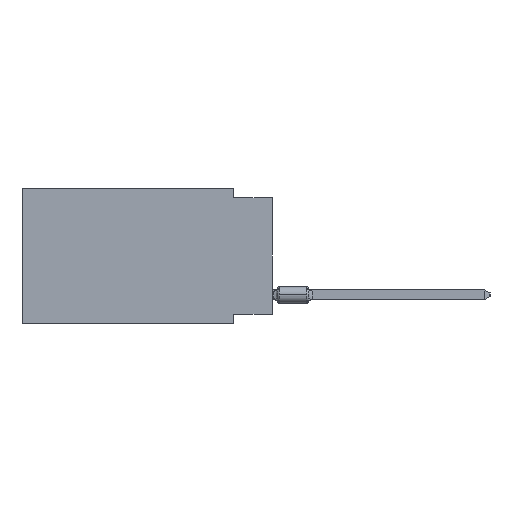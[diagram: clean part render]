
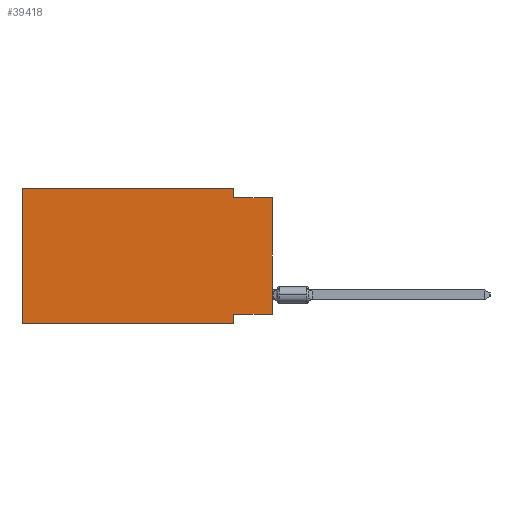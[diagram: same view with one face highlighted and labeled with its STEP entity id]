
A CAD part, left-side view. The second image highlights one B-rep face of the part: STEP entity #39418.
In plain terms, the highlighted planar face has unit normal (-1, 0, 0).
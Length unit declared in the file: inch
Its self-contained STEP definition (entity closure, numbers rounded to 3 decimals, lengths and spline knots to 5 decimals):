
#1447 = VERTEX_POINT ( 'NONE', #66218 ) ;
#1504 = LINE ( 'NONE', #48722, #43938 ) ;
#1848 = FACE_OUTER_BOUND ( 'NONE', #68202, .T. ) ;
#2278 = CARTESIAN_POINT ( 'NONE',  ( 0., 0.645, 0. ) ) ;
#4499 = VECTOR ( 'NONE', #53500, 39.37008 ) ;
#5767 = CARTESIAN_POINT ( 'NONE',  ( 0., 0.1, -0.35 ) ) ;
#6463 = ORIENTED_EDGE ( 'NONE', *, *, #48289, .T. ) ;
#7858 = DIRECTION ( 'NONE',  ( 0., 0., 1. ) ) ;
#8450 = PLANE ( 'NONE',  #67517 ) ;
#8498 = ORIENTED_EDGE ( 'NONE', *, *, #52676, .F. ) ;
#10071 = DIRECTION ( 'NONE',  ( 0., 0., -1. ) ) ;
#10268 = ORIENTED_EDGE ( 'NONE', *, *, #32074, .T. ) ;
#10393 = VERTEX_POINT ( 'NONE', #55037 ) ;
#10540 = VERTEX_POINT ( 'NONE', #61678 ) ;
#10897 = VECTOR ( 'NONE', #47799, 39.37008 ) ;
#11428 = ORIENTED_EDGE ( 'NONE', *, *, #39035, .F. ) ;
#11627 = VECTOR ( 'NONE', #7858, 39.37008 ) ;
#12656 = DIRECTION ( 'NONE',  ( 0., 0., -1. ) ) ;
#13071 = VERTEX_POINT ( 'NONE', #23697 ) ;
#13671 = VERTEX_POINT ( 'NONE', #41412 ) ;
#16174 = LINE ( 'NONE', #58866, #17674 ) ;
#16407 = LINE ( 'NONE', #21311, #4499 ) ;
#17674 = VECTOR ( 'NONE', #25656, 39.37008 ) ;
#18840 = VECTOR ( 'NONE', #66236, 39.37008 ) ;
#21066 = ORIENTED_EDGE ( 'NONE', *, *, #36596, .F. ) ;
#21311 = CARTESIAN_POINT ( 'NONE',  ( 0., 0.645, 0. ) ) ;
#22012 = ORIENTED_EDGE ( 'NONE', *, *, #31696, .F. ) ;
#22060 = VECTOR ( 'NONE', #10071, 39.37008 ) ;
#22874 = LINE ( 'NONE', #61347, #18840 ) ;
#23515 = DIRECTION ( 'NONE',  ( 1., 0., 0. ) ) ;
#23697 = CARTESIAN_POINT ( 'NONE',  ( 0., 0.645, 0. ) ) ;
#25148 = VERTEX_POINT ( 'NONE', #34163 ) ;
#25656 = DIRECTION ( 'NONE',  ( 0., 0., 1. ) ) ;
#26456 = CARTESIAN_POINT ( 'NONE',  ( 0., 0., -0.025 ) ) ;
#27095 = DIRECTION ( 'NONE',  ( 0., 0., -1. ) ) ;
#27178 = CARTESIAN_POINT ( 'NONE',  ( 0., 0.1, 0. ) ) ;
#29430 = CARTESIAN_POINT ( 'NONE',  ( 0., 0.645, 0. ) ) ;
#29437 = EDGE_CURVE ( 'NONE', #10540, #13671, #48176, .T. ) ;
#31696 = EDGE_CURVE ( 'NONE', #33998, #10393, #32355, .T. ) ;
#31703 = LINE ( 'NONE', #26456, #10897 ) ;
#32074 = EDGE_CURVE ( 'NONE', #1447, #40912, #16174, .T. ) ;
#32355 = LINE ( 'NONE', #5767, #36587 ) ;
#32447 = CARTESIAN_POINT ( 'NONE',  ( 0., 0., -0.025 ) ) ;
#33998 = VERTEX_POINT ( 'NONE', #57048 ) ;
#34163 = CARTESIAN_POINT ( 'NONE',  ( 0., 0.645, -0.35 ) ) ;
#36587 = VECTOR ( 'NONE', #27095, 39.37008 ) ;
#36596 = EDGE_CURVE ( 'NONE', #1447, #33998, #1504, .T. ) ;
#39035 = EDGE_CURVE ( 'NONE', #25148, #13071, #55774, .T. ) ;
#39418 = ADVANCED_FACE ( 'NONE', ( #1848 ), #8450, .F. ) ;
#40912 = VERTEX_POINT ( 'NONE', #32447 ) ;
#41412 = CARTESIAN_POINT ( 'NONE',  ( 0., 0.1, -0.025 ) ) ;
#42070 = ORIENTED_EDGE ( 'NONE', *, *, #29437, .F. ) ;
#43938 = VECTOR ( 'NONE', #65517, 39.37008 ) ;
#47799 = DIRECTION ( 'NONE',  ( 0., -1., 0. ) ) ;
#48176 = LINE ( 'NONE', #27178, #22060 ) ;
#48289 = EDGE_CURVE ( 'NONE', #25148, #10393, #22874, .T. ) ;
#48722 = CARTESIAN_POINT ( 'NONE',  ( 0., 0., -0.325 ) ) ;
#52676 = EDGE_CURVE ( 'NONE', #13671, #40912, #31703, .T. ) ;
#53500 = DIRECTION ( 'NONE',  ( 0., -1., 0. ) ) ;
#55037 = CARTESIAN_POINT ( 'NONE',  ( 0., 0.1, -0.35 ) ) ;
#55774 = LINE ( 'NONE', #2278, #11627 ) ;
#57048 = CARTESIAN_POINT ( 'NONE',  ( 0., 0.1, -0.325 ) ) ;
#58866 = CARTESIAN_POINT ( 'NONE',  ( 0., 0., 0. ) ) ;
#61347 = CARTESIAN_POINT ( 'NONE',  ( 0., 0.645, -0.35 ) ) ;
#61678 = CARTESIAN_POINT ( 'NONE',  ( 0., 0.1, 0. ) ) ;
#61730 = ORIENTED_EDGE ( 'NONE', *, *, #62682, .F. ) ;
#62682 = EDGE_CURVE ( 'NONE', #13071, #10540, #16407, .T. ) ;
#65517 = DIRECTION ( 'NONE',  ( 0., 1., 0. ) ) ;
#66218 = CARTESIAN_POINT ( 'NONE',  ( 0., 0., -0.325 ) ) ;
#66236 = DIRECTION ( 'NONE',  ( 0., -1., 0. ) ) ;
#67517 = AXIS2_PLACEMENT_3D ( 'NONE', #29430, #23515, #12656 ) ;
#68202 = EDGE_LOOP ( 'NONE', ( #10268, #8498, #42070, #61730, #11428, #6463, #22012, #21066 ) ) ;
